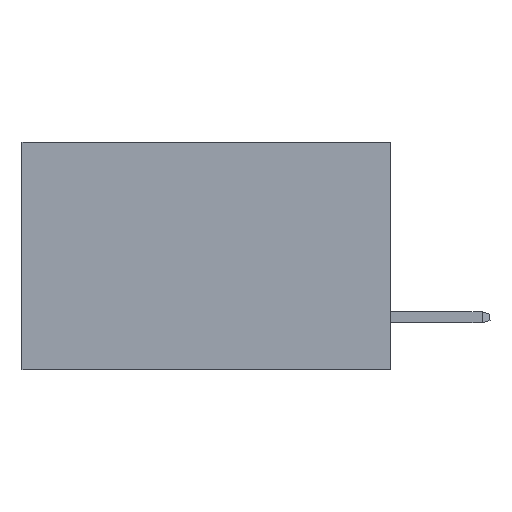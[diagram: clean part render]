
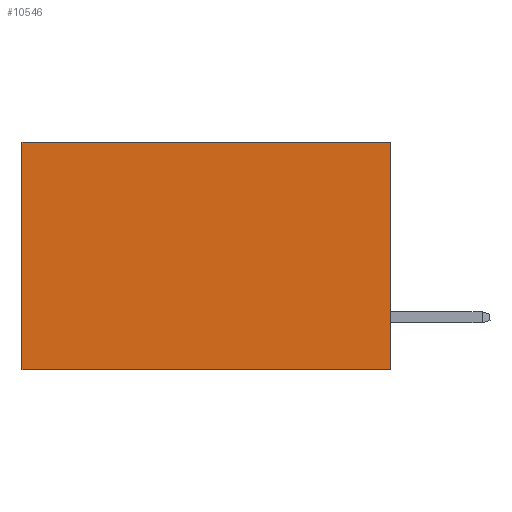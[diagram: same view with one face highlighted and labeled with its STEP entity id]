
A CAD part, left-side view. The second image highlights one B-rep face of the part: STEP entity #10546.
In plain terms, the highlighted planar face has unit normal (-1, 0, 0).
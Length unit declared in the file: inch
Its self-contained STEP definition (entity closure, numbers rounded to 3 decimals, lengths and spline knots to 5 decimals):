
#752 = ORIENTED_EDGE ( 'NONE', *, *, #6059, .F. ) ;
#1326 = DIRECTION ( 'NONE',  ( 0., 0., -1. ) ) ;
#3703 = VECTOR ( 'NONE', #1326, 39.37008 ) ;
#4177 = ORIENTED_EDGE ( 'NONE', *, *, #14933, .T. ) ;
#4883 = DIRECTION ( 'NONE',  ( 1., 0., 0. ) ) ;
#5438 = EDGE_LOOP ( 'NONE', ( #9456, #12009, #752, #4177 ) ) ;
#6059 = EDGE_CURVE ( 'NONE', #10003, #7113, #7805, .T. ) ;
#6574 = DIRECTION ( 'NONE',  ( 0., 0., -1. ) ) ;
#6788 = CARTESIAN_POINT ( 'NONE',  ( 0.2875, 0.6, 0. ) ) ;
#7113 = VERTEX_POINT ( 'NONE', #12969 ) ;
#7437 = VECTOR ( 'NONE', #12843, 39.37008 ) ;
#7710 = LINE ( 'NONE', #14325, #14155 ) ;
#7805 = LINE ( 'NONE', #9620, #3703 ) ;
#7807 = CARTESIAN_POINT ( 'NONE',  ( 0.2875, 0., 0. ) ) ;
#7821 = AXIS2_PLACEMENT_3D ( 'NONE', #10248, #4883, #14044 ) ;
#8347 = CARTESIAN_POINT ( 'NONE',  ( 0.2875, 0.6, -0.37 ) ) ;
#9456 = ORIENTED_EDGE ( 'NONE', *, *, #13730, .T. ) ;
#9620 = CARTESIAN_POINT ( 'NONE',  ( 0.2875, 0., 0. ) ) ;
#10003 = VERTEX_POINT ( 'NONE', #7807 ) ;
#10163 = VERTEX_POINT ( 'NONE', #6788 ) ;
#10248 = CARTESIAN_POINT ( 'NONE',  ( 0.2875, 0., 0. ) ) ;
#10546 = ADVANCED_FACE ( 'NONE', ( #11563 ), #12815, .F. ) ;
#11158 = LINE ( 'NONE', #13757, #13365 ) ;
#11353 = LINE ( 'NONE', #16485, #7437 ) ;
#11563 = FACE_OUTER_BOUND ( 'NONE', #5438, .T. ) ;
#12009 = ORIENTED_EDGE ( 'NONE', *, *, #15073, .F. ) ;
#12520 = DIRECTION ( 'NONE',  ( 0., 1., 0. ) ) ;
#12815 = PLANE ( 'NONE',  #7821 ) ;
#12843 = DIRECTION ( 'NONE',  ( 0., 1., 0. ) ) ;
#12969 = CARTESIAN_POINT ( 'NONE',  ( 0.2875, 0., -0.37 ) ) ;
#13365 = VECTOR ( 'NONE', #12520, 39.37008 ) ;
#13730 = EDGE_CURVE ( 'NONE', #10163, #15396, #7710, .T. ) ;
#13757 = CARTESIAN_POINT ( 'NONE',  ( 0.2875, 0., 0. ) ) ;
#14044 = DIRECTION ( 'NONE',  ( 0., 0., -1. ) ) ;
#14155 = VECTOR ( 'NONE', #6574, 39.37008 ) ;
#14325 = CARTESIAN_POINT ( 'NONE',  ( 0.2875, 0.6, 0. ) ) ;
#14933 = EDGE_CURVE ( 'NONE', #10003, #10163, #11158, .T. ) ;
#15073 = EDGE_CURVE ( 'NONE', #7113, #15396, #11353, .T. ) ;
#15396 = VERTEX_POINT ( 'NONE', #8347 ) ;
#16485 = CARTESIAN_POINT ( 'NONE',  ( 0.2875, 0., -0.37 ) ) ;
